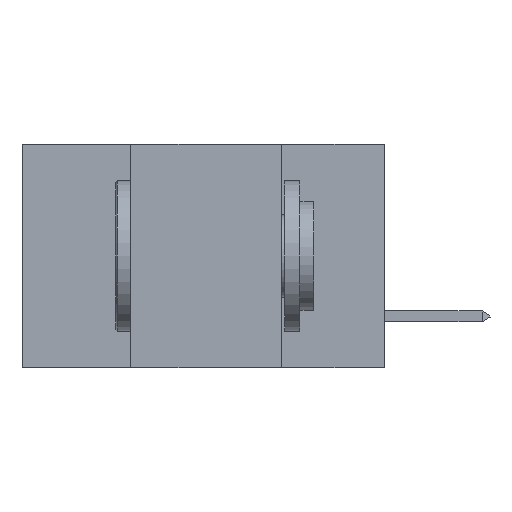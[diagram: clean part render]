
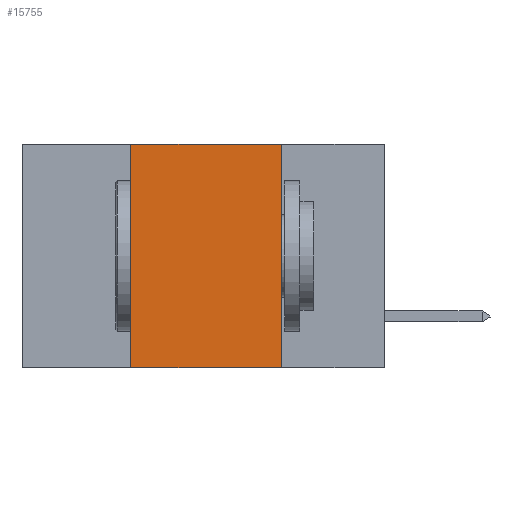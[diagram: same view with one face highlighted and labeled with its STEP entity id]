
A CAD part, left-side view. The second image highlights one B-rep face of the part: STEP entity #15755.
In plain terms, the highlighted planar face has unit normal (-1, 0, 0).
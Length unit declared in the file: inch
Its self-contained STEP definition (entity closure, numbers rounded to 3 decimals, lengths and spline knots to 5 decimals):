
#518 = VECTOR ( 'NONE', #13212, 39.37008 ) ;
#714 = ORIENTED_EDGE ( 'NONE', *, *, #18846, .F. ) ;
#905 = CARTESIAN_POINT ( 'NONE',  ( 0., 0.17, 0. ) ) ;
#1216 = CARTESIAN_POINT ( 'NONE',  ( 0., 0.6, 0. ) ) ;
#1632 = CARTESIAN_POINT ( 'NONE',  ( 0., 0.6, -0.37 ) ) ;
#2461 = VECTOR ( 'NONE', #5673, 39.37008 ) ;
#2711 = CARTESIAN_POINT ( 'NONE',  ( 0., 0.17, 0. ) ) ;
#4302 = AXIS2_PLACEMENT_3D ( 'NONE', #20503, #15364, #7283 ) ;
#5673 = DIRECTION ( 'NONE',  ( 0., 0., -1. ) ) ;
#7283 = DIRECTION ( 'NONE',  ( 0., 0., -1. ) ) ;
#7380 = VERTEX_POINT ( 'NONE', #16207 ) ;
#7385 = CARTESIAN_POINT ( 'NONE',  ( 0., 0.42, -0.37 ) ) ;
#8449 = LINE ( 'NONE', #11345, #12555 ) ;
#9290 = ORIENTED_EDGE ( 'NONE', *, *, #13995, .F. ) ;
#9311 = LINE ( 'NONE', #1632, #518 ) ;
#9557 = DIRECTION ( 'NONE',  ( 0., 0., 1. ) ) ;
#9912 = LINE ( 'NONE', #1216, #17949 ) ;
#11345 = CARTESIAN_POINT ( 'NONE',  ( 0., 0.42, 0. ) ) ;
#11458 = VERTEX_POINT ( 'NONE', #7385 ) ;
#12555 = VECTOR ( 'NONE', #9557, 39.37008 ) ;
#13212 = DIRECTION ( 'NONE',  ( 0., -1., 0. ) ) ;
#13466 = EDGE_LOOP ( 'NONE', ( #16750, #9290, #714, #17095 ) ) ;
#13995 = EDGE_CURVE ( 'NONE', #16256, #19751, #9912, .T. ) ;
#15060 = CARTESIAN_POINT ( 'NONE',  ( 0., 0.42, 0. ) ) ;
#15286 = FACE_OUTER_BOUND ( 'NONE', #13466, .T. ) ;
#15288 = PLANE ( 'NONE',  #4302 ) ;
#15364 = DIRECTION ( 'NONE',  ( 1., 0., 0. ) ) ;
#15755 = ADVANCED_FACE ( 'NONE', ( #15286 ), #15288, .F. ) ;
#16207 = CARTESIAN_POINT ( 'NONE',  ( 0., 0.17, -0.37 ) ) ;
#16256 = VERTEX_POINT ( 'NONE', #15060 ) ;
#16750 = ORIENTED_EDGE ( 'NONE', *, *, #21179, .F. ) ;
#16859 = EDGE_CURVE ( 'NONE', #11458, #7380, #9311, .T. ) ;
#17095 = ORIENTED_EDGE ( 'NONE', *, *, #16859, .T. ) ;
#17565 = DIRECTION ( 'NONE',  ( 0., -1., 0. ) ) ;
#17949 = VECTOR ( 'NONE', #17565, 39.37008 ) ;
#18846 = EDGE_CURVE ( 'NONE', #11458, #16256, #8449, .T. ) ;
#19751 = VERTEX_POINT ( 'NONE', #905 ) ;
#20281 = LINE ( 'NONE', #2711, #2461 ) ;
#20503 = CARTESIAN_POINT ( 'NONE',  ( 0., 0.6, 0. ) ) ;
#21179 = EDGE_CURVE ( 'NONE', #19751, #7380, #20281, .T. ) ;
